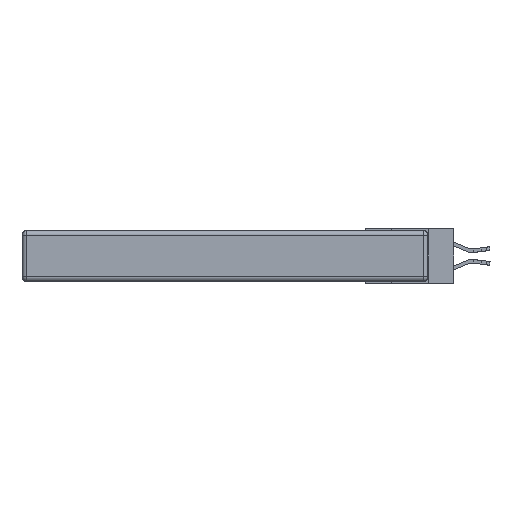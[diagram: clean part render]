
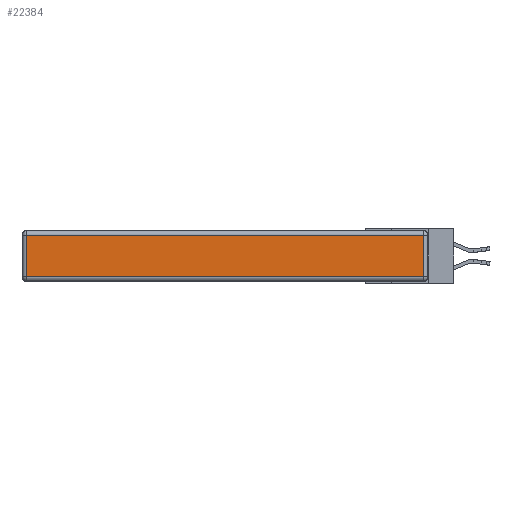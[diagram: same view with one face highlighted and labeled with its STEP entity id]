
A CAD part, left-side view. The second image highlights one B-rep face of the part: STEP entity #22384.
In plain terms, the highlighted planar face has unit normal (-1, 0, 0).
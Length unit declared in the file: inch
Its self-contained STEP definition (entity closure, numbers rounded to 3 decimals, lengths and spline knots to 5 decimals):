
#302 = PLANE ( 'NONE',  #2897 ) ;
#440 = DIRECTION ( 'NONE',  ( 0., -1., 0. ) ) ;
#542 = EDGE_CURVE ( 'NONE', #24662, #3776, #7670, .T. ) ;
#2423 = DIRECTION ( 'NONE',  ( -1., 0., 0. ) ) ;
#2864 = DIRECTION ( 'NONE',  ( 0., 0., -1. ) ) ;
#2897 = AXIS2_PLACEMENT_3D ( 'NONE', #4833, #2423, #11531 ) ;
#3776 = VERTEX_POINT ( 'NONE', #20522 ) ;
#4268 = EDGE_CURVE ( 'NONE', #3776, #11762, #16765, .T. ) ;
#4833 = CARTESIAN_POINT ( 'NONE',  ( 0., 0., -0.343 ) ) ;
#5163 = ORIENTED_EDGE ( 'NONE', *, *, #21350, .T. ) ;
#5281 = VECTOR ( 'NONE', #12872, 39.37008 ) ;
#5973 = FACE_OUTER_BOUND ( 'NONE', #12798, .T. ) ;
#6971 = ORIENTED_EDGE ( 'NONE', *, *, #542, .T. ) ;
#7325 = VECTOR ( 'NONE', #440, 39.37008 ) ;
#7612 = VERTEX_POINT ( 'NONE', #19451 ) ;
#7670 = LINE ( 'NONE', #11473, #7325 ) ;
#8211 = CARTESIAN_POINT ( 'NONE',  ( 0., 2.75, -0.03 ) ) ;
#9966 = ORIENTED_EDGE ( 'NONE', *, *, #4268, .T. ) ;
#10961 = VECTOR ( 'NONE', #2864, 39.37008 ) ;
#11473 = CARTESIAN_POINT ( 'NONE',  ( 0., 0., -0.313 ) ) ;
#11531 = DIRECTION ( 'NONE',  ( 0., 0., 1. ) ) ;
#11762 = VERTEX_POINT ( 'NONE', #18085 ) ;
#11999 = ORIENTED_EDGE ( 'NONE', *, *, #20330, .T. ) ;
#12798 = EDGE_LOOP ( 'NONE', ( #6971, #9966, #11999, #5163 ) ) ;
#12872 = DIRECTION ( 'NONE',  ( 0., 0., 1. ) ) ;
#14444 = LINE ( 'NONE', #16330, #10961 ) ;
#14880 = LINE ( 'NONE', #8211, #20415 ) ;
#16330 = CARTESIAN_POINT ( 'NONE',  ( 0., 2.72, -0.343 ) ) ;
#16765 = LINE ( 'NONE', #17166, #5281 ) ;
#17166 = CARTESIAN_POINT ( 'NONE',  ( 0., 0.03, -0.343 ) ) ;
#18085 = CARTESIAN_POINT ( 'NONE',  ( 0., 0.03, -0.03 ) ) ;
#19451 = CARTESIAN_POINT ( 'NONE',  ( 0., 2.72, -0.03 ) ) ;
#20330 = EDGE_CURVE ( 'NONE', #11762, #7612, #14880, .T. ) ;
#20415 = VECTOR ( 'NONE', #21711, 39.37008 ) ;
#20522 = CARTESIAN_POINT ( 'NONE',  ( 0., 0.03, -0.313 ) ) ;
#20945 = CARTESIAN_POINT ( 'NONE',  ( 0., 2.72, -0.313 ) ) ;
#21350 = EDGE_CURVE ( 'NONE', #7612, #24662, #14444, .T. ) ;
#21711 = DIRECTION ( 'NONE',  ( 0., 1., 0. ) ) ;
#22384 = ADVANCED_FACE ( 'NONE', ( #5973 ), #302, .T. ) ;
#24662 = VERTEX_POINT ( 'NONE', #20945 ) ;
